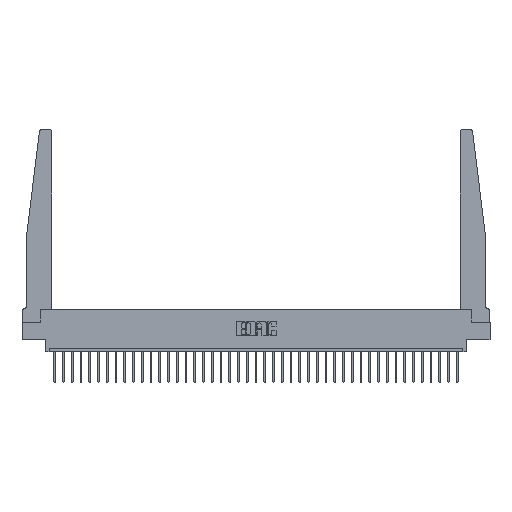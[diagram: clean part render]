
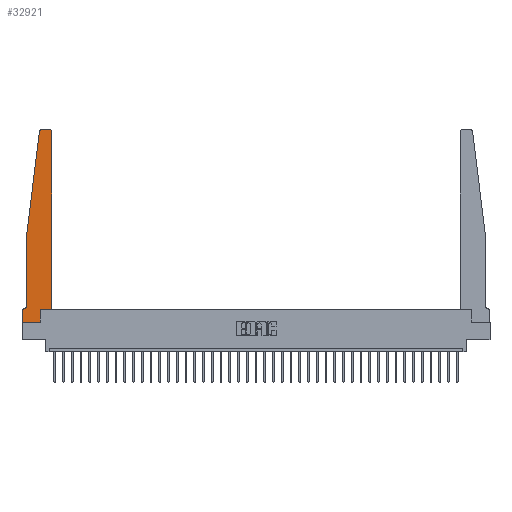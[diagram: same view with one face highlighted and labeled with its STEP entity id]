
A CAD part, top view. The second image highlights one B-rep face of the part: STEP entity #32921.
In plain terms, the highlighted planar face has unit normal (0, 0, 1).
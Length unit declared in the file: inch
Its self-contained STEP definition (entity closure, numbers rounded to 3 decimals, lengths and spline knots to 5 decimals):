
#30 = CARTESIAN_POINT ( 'NONE',  ( 0.2605, 0., 0.37 ) ) ;
#174 = ORIENTED_EDGE ( 'NONE', *, *, #5093, .T. ) ;
#181 = VERTEX_POINT ( 'NONE', #20113 ) ;
#866 = CARTESIAN_POINT ( 'NONE',  ( 0.395, 2.75, 0.37 ) ) ;
#2632 = EDGE_CURVE ( 'NONE', #21206, #14023, #3533, .T. ) ;
#3533 = LINE ( 'NONE', #22962, #4731 ) ;
#3779 = AXIS2_PLACEMENT_3D ( 'NONE', #4304, #27756, #22491 ) ;
#4304 = CARTESIAN_POINT ( 'NONE',  ( 0.015, 0.2375, 0.37 ) ) ;
#4458 = AXIS2_PLACEMENT_3D ( 'NONE', #27759, #4873, #12556 ) ;
#4731 = VECTOR ( 'NONE', #14838, 39.37008 ) ;
#4873 = DIRECTION ( 'NONE',  ( 0., 0., 1. ) ) ;
#4898 = VERTEX_POINT ( 'NONE', #6398 ) ;
#5093 = EDGE_CURVE ( 'NONE', #22692, #21206, #9114, .T. ) ;
#5261 = ORIENTED_EDGE ( 'NONE', *, *, #28876, .T. ) ;
#5335 = LINE ( 'NONE', #29264, #25892 ) ;
#5839 = CARTESIAN_POINT ( 'NONE',  ( 0., 0., 0.37 ) ) ;
#6361 = ORIENTED_EDGE ( 'NONE', *, *, #14060, .T. ) ;
#6398 = CARTESIAN_POINT ( 'NONE',  ( 0.065, 0.2375, 0.37 ) ) ;
#7140 = PLANE ( 'NONE',  #15405 ) ;
#7184 = CARTESIAN_POINT ( 'NONE',  ( 0., 0.1875, 0.37 ) ) ;
#7882 = LINE ( 'NONE', #16627, #9965 ) ;
#7973 = DIRECTION ( 'NONE',  ( 0., -1., 0. ) ) ;
#8053 = CARTESIAN_POINT ( 'NONE',  ( 0.015, 0.1875, 0.37 ) ) ;
#8325 = CIRCLE ( 'NONE', #4458, 0.03 ) ;
#8535 = ORIENTED_EDGE ( 'NONE', *, *, #24533, .T. ) ;
#8623 = EDGE_LOOP ( 'NONE', ( #18110, #19870, #8944, #30070, #8535, #6361, #174, #26249, #12877, #5261, #30493, #27198 ) ) ;
#8752 = DIRECTION ( 'NONE',  ( -1., 0., 0. ) ) ;
#8795 = VERTEX_POINT ( 'NONE', #8053 ) ;
#8944 = ORIENTED_EDGE ( 'NONE', *, *, #12133, .T. ) ;
#9114 = LINE ( 'NONE', #14870, #30110 ) ;
#9198 = DIRECTION ( 'NONE',  ( 0., 0., 1. ) ) ;
#9965 = VECTOR ( 'NONE', #11575, 39.37008 ) ;
#10668 = LINE ( 'NONE', #25755, #30421 ) ;
#10799 = EDGE_CURVE ( 'NONE', #15679, #22230, #29782, .T. ) ;
#11575 = DIRECTION ( 'NONE',  ( -0.122, -0.992, 0. ) ) ;
#11856 = CARTESIAN_POINT ( 'NONE',  ( 0.25, 2.75, 0.37 ) ) ;
#12133 = EDGE_CURVE ( 'NONE', #22230, #181, #7882, .T. ) ;
#12249 = AXIS2_PLACEMENT_3D ( 'NONE', #27288, #9198, #32608 ) ;
#12325 = EDGE_CURVE ( 'NONE', #29372, #24960, #8325, .T. ) ;
#12345 = DIRECTION ( 'NONE',  ( 0., 0., 1. ) ) ;
#12556 = DIRECTION ( 'NONE',  ( 1., 0., 0. ) ) ;
#12877 = ORIENTED_EDGE ( 'NONE', *, *, #19504, .T. ) ;
#14023 = VERTEX_POINT ( 'NONE', #30 ) ;
#14060 = EDGE_CURVE ( 'NONE', #8795, #22692, #5335, .T. ) ;
#14096 = LINE ( 'NONE', #32896, #18953 ) ;
#14838 = DIRECTION ( 'NONE',  ( 1., 0., 0. ) ) ;
#14870 = CARTESIAN_POINT ( 'NONE',  ( 0., 0., 0.37 ) ) ;
#15405 = AXIS2_PLACEMENT_3D ( 'NONE', #25162, #12345, #30364 ) ;
#15493 = CARTESIAN_POINT ( 'NONE',  ( 0.425, 0.18, 0.37 ) ) ;
#15679 = VERTEX_POINT ( 'NONE', #27591 ) ;
#15730 = DIRECTION ( 'NONE',  ( 0., 1., 0. ) ) ;
#16627 = CARTESIAN_POINT ( 'NONE',  ( 0.065, 1.25, 0.37 ) ) ;
#17250 = CARTESIAN_POINT ( 'NONE',  ( 0.425, 0.18, 0.37 ) ) ;
#17276 = DIRECTION ( 'NONE',  ( 0., -1., 0. ) ) ;
#17353 = DIRECTION ( 'NONE',  ( -1., 0., 0. ) ) ;
#17719 = CARTESIAN_POINT ( 'NONE',  ( 0.24675, 2.72367, 0.37 ) ) ;
#18110 = ORIENTED_EDGE ( 'NONE', *, *, #29293, .T. ) ;
#18333 = DIRECTION ( 'NONE',  ( 1., 0., 0. ) ) ;
#18953 = VECTOR ( 'NONE', #17276, 39.37008 ) ;
#19146 = EDGE_CURVE ( 'NONE', #22563, #29372, #32407, .T. ) ;
#19504 = EDGE_CURVE ( 'NONE', #14023, #32648, #10668, .T. ) ;
#19870 = ORIENTED_EDGE ( 'NONE', *, *, #10799, .T. ) ;
#20113 = CARTESIAN_POINT ( 'NONE',  ( 0.065, 1.25, 0.37 ) ) ;
#21206 = VERTEX_POINT ( 'NONE', #5839 ) ;
#21459 = LINE ( 'NONE', #15493, #32305 ) ;
#21850 = LINE ( 'NONE', #11856, #33098 ) ;
#22230 = VERTEX_POINT ( 'NONE', #17719 ) ;
#22491 = DIRECTION ( 'NONE',  ( -1., 0., 0. ) ) ;
#22563 = VERTEX_POINT ( 'NONE', #27086 ) ;
#22692 = VERTEX_POINT ( 'NONE', #7184 ) ;
#22758 = DIRECTION ( 'NONE',  ( 0., 1., 0. ) ) ;
#22816 = FACE_OUTER_BOUND ( 'NONE', #8623, .T. ) ;
#22962 = CARTESIAN_POINT ( 'NONE',  ( 0., 0., 0.37 ) ) ;
#22968 = CIRCLE ( 'NONE', #3779, 0.05 ) ;
#24533 = EDGE_CURVE ( 'NONE', #4898, #8795, #22968, .T. ) ;
#24960 = VERTEX_POINT ( 'NONE', #866 ) ;
#25162 = CARTESIAN_POINT ( 'NONE',  ( 0., 0.1875, 0.37 ) ) ;
#25755 = CARTESIAN_POINT ( 'NONE',  ( 0.2605, 0.18, 0.37 ) ) ;
#25892 = VECTOR ( 'NONE', #8752, 39.37008 ) ;
#26192 = CARTESIAN_POINT ( 'NONE',  ( 0.2605, 0.18, 0.37 ) ) ;
#26249 = ORIENTED_EDGE ( 'NONE', *, *, #2632, .T. ) ;
#27086 = CARTESIAN_POINT ( 'NONE',  ( 0.425, 0.18, 0.37 ) ) ;
#27198 = ORIENTED_EDGE ( 'NONE', *, *, #12325, .T. ) ;
#27288 = CARTESIAN_POINT ( 'NONE',  ( 0.27653, 2.72, 0.37 ) ) ;
#27333 = CARTESIAN_POINT ( 'NONE',  ( 0.425, 2.72, 0.37 ) ) ;
#27591 = CARTESIAN_POINT ( 'NONE',  ( 0.27653, 2.75, 0.37 ) ) ;
#27756 = DIRECTION ( 'NONE',  ( 0., 0., -1. ) ) ;
#27759 = CARTESIAN_POINT ( 'NONE',  ( 0.395, 2.72, 0.37 ) ) ;
#27993 = VECTOR ( 'NONE', #22758, 39.37008 ) ;
#28876 = EDGE_CURVE ( 'NONE', #32648, #22563, #21459, .T. ) ;
#29264 = CARTESIAN_POINT ( 'NONE',  ( 0.065, 0.1875, 0.37 ) ) ;
#29293 = EDGE_CURVE ( 'NONE', #24960, #15679, #21850, .T. ) ;
#29372 = VERTEX_POINT ( 'NONE', #27333 ) ;
#29782 = CIRCLE ( 'NONE', #12249, 0.03 ) ;
#30070 = ORIENTED_EDGE ( 'NONE', *, *, #30726, .T. ) ;
#30110 = VECTOR ( 'NONE', #7973, 39.37008 ) ;
#30364 = DIRECTION ( 'NONE',  ( 1., 0., 0. ) ) ;
#30421 = VECTOR ( 'NONE', #15730, 39.37008 ) ;
#30493 = ORIENTED_EDGE ( 'NONE', *, *, #19146, .T. ) ;
#30726 = EDGE_CURVE ( 'NONE', #181, #4898, #14096, .T. ) ;
#32305 = VECTOR ( 'NONE', #18333, 39.37008 ) ;
#32407 = LINE ( 'NONE', #17250, #27993 ) ;
#32608 = DIRECTION ( 'NONE',  ( 1., 0., 0. ) ) ;
#32648 = VERTEX_POINT ( 'NONE', #26192 ) ;
#32896 = CARTESIAN_POINT ( 'NONE',  ( 0.065, 1.25, 0.37 ) ) ;
#32921 = ADVANCED_FACE ( 'NONE', ( #22816 ), #7140, .T. ) ;
#33098 = VECTOR ( 'NONE', #17353, 39.37008 ) ;
